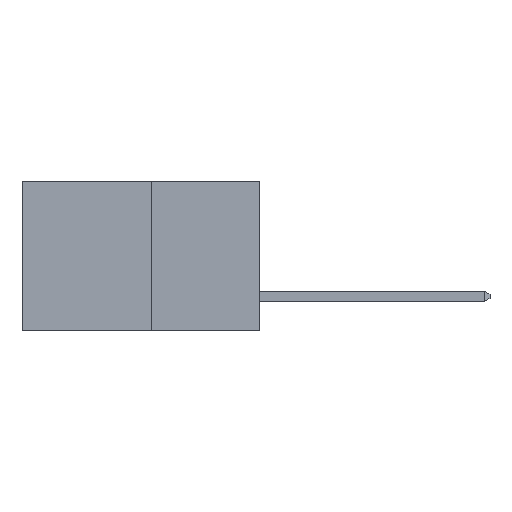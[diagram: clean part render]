
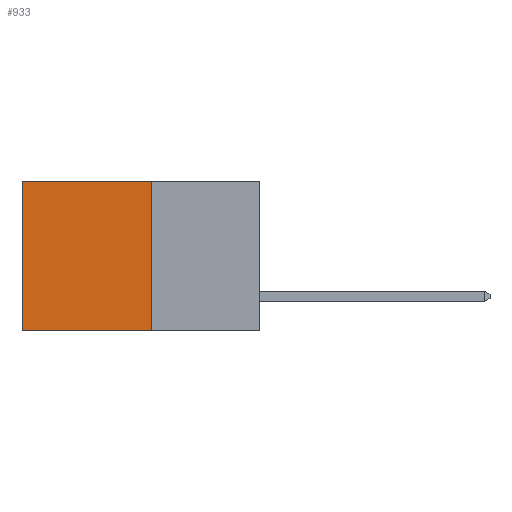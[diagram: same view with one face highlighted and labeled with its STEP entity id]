
A CAD part, left-side view. The second image highlights one B-rep face of the part: STEP entity #933.
In plain terms, the highlighted planar face has unit normal (-1, 0, 0).
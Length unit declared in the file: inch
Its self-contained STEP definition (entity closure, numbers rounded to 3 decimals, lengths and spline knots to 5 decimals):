
#77 = DIRECTION ( 'NONE',  ( 0., 0., -1. ) ) ;
#119 = VERTEX_POINT ( 'NONE', #6469 ) ;
#394 = VECTOR ( 'NONE', #8095, 39.37008 ) ;
#511 = VECTOR ( 'NONE', #5214, 39.37008 ) ;
#585 = CARTESIAN_POINT ( 'NONE',  ( 0.277, 0.59, 0. ) ) ;
#862 = DIRECTION ( 'NONE',  ( 1., 0., 0. ) ) ;
#933 = ADVANCED_FACE ( 'NONE', ( #2905 ), #1349, .F. ) ;
#973 = EDGE_CURVE ( 'NONE', #4062, #5602, #7838, .T. ) ;
#1162 = ORIENTED_EDGE ( 'NONE', *, *, #973, .F. ) ;
#1349 = PLANE ( 'NONE',  #7081 ) ;
#1357 = CARTESIAN_POINT ( 'NONE',  ( 0.277, 0.27, -0.37 ) ) ;
#2128 = LINE ( 'NONE', #8233, #394 ) ;
#2468 = LINE ( 'NONE', #5243, #511 ) ;
#2620 = EDGE_CURVE ( 'NONE', #4003, #119, #2128, .T. ) ;
#2905 = FACE_OUTER_BOUND ( 'NONE', #6634, .T. ) ;
#2953 = ORIENTED_EDGE ( 'NONE', *, *, #7589, .T. ) ;
#4003 = VERTEX_POINT ( 'NONE', #585 ) ;
#4062 = VERTEX_POINT ( 'NONE', #4548 ) ;
#4161 = DIRECTION ( 'NONE',  ( 0., 0., -1. ) ) ;
#4425 = VECTOR ( 'NONE', #6021, 39.37008 ) ;
#4548 = CARTESIAN_POINT ( 'NONE',  ( 0.277, 0.27, 0. ) ) ;
#5214 = DIRECTION ( 'NONE',  ( 0., 1., 0. ) ) ;
#5243 = CARTESIAN_POINT ( 'NONE',  ( 0.277, 0.27, 0. ) ) ;
#5602 = VERTEX_POINT ( 'NONE', #5844 ) ;
#5844 = CARTESIAN_POINT ( 'NONE',  ( 0.277, 0.27, -0.37 ) ) ;
#5890 = LINE ( 'NONE', #6023, #4425 ) ;
#5996 = VECTOR ( 'NONE', #4161, 39.37008 ) ;
#6021 = DIRECTION ( 'NONE',  ( 0., 1., 0. ) ) ;
#6023 = CARTESIAN_POINT ( 'NONE',  ( 0.277, 0.27, -0.37 ) ) ;
#6249 = ORIENTED_EDGE ( 'NONE', *, *, #2620, .T. ) ;
#6469 = CARTESIAN_POINT ( 'NONE',  ( 0.277, 0.59, -0.37 ) ) ;
#6634 = EDGE_LOOP ( 'NONE', ( #6249, #7872, #1162, #2953 ) ) ;
#7081 = AXIS2_PLACEMENT_3D ( 'NONE', #1357, #862, #77 ) ;
#7343 = EDGE_CURVE ( 'NONE', #5602, #119, #5890, .T. ) ;
#7589 = EDGE_CURVE ( 'NONE', #4062, #4003, #2468, .T. ) ;
#7838 = LINE ( 'NONE', #8211, #5996 ) ;
#7872 = ORIENTED_EDGE ( 'NONE', *, *, #7343, .F. ) ;
#8095 = DIRECTION ( 'NONE',  ( 0., 0., -1. ) ) ;
#8211 = CARTESIAN_POINT ( 'NONE',  ( 0.277, 0.27, -0.37 ) ) ;
#8233 = CARTESIAN_POINT ( 'NONE',  ( 0.277, 0.59, -0.37 ) ) ;
